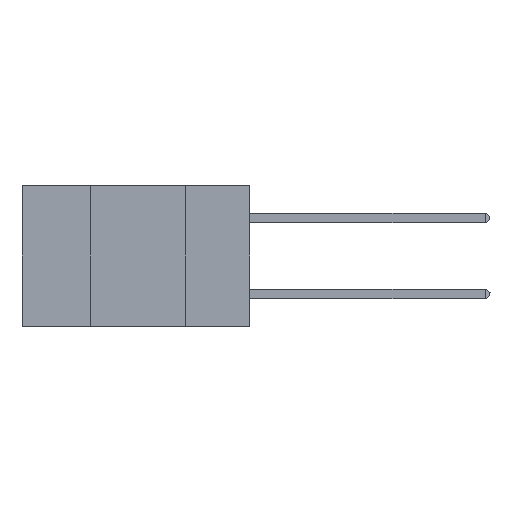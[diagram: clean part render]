
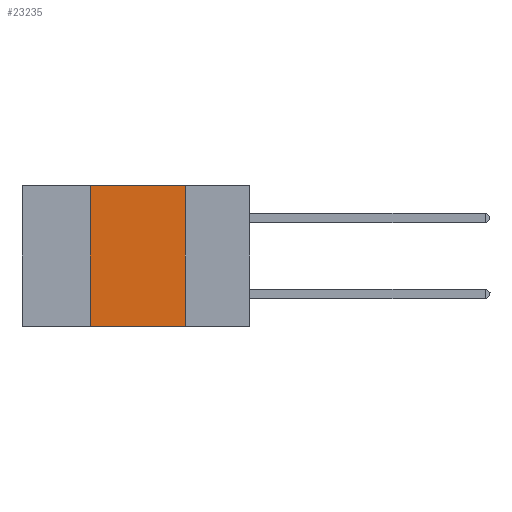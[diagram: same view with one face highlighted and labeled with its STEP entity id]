
A CAD part, left-side view. The second image highlights one B-rep face of the part: STEP entity #23235.
In plain terms, the highlighted planar face has unit normal (-1, 0, 0).
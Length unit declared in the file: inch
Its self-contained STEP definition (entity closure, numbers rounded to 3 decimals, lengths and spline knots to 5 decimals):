
#837 = CARTESIAN_POINT ( 'NONE',  ( 0., 0.42, -0.37 ) ) ;
#2333 = ORIENTED_EDGE ( 'NONE', *, *, #28997, .F. ) ;
#3113 = CARTESIAN_POINT ( 'NONE',  ( 0., 0.6, 0. ) ) ;
#4194 = VERTEX_POINT ( 'NONE', #9329 ) ;
#6163 = PLANE ( 'NONE',  #11271 ) ;
#8453 = ORIENTED_EDGE ( 'NONE', *, *, #9133, .T. ) ;
#9133 = EDGE_CURVE ( 'NONE', #16086, #14528, #12765, .T. ) ;
#9329 = CARTESIAN_POINT ( 'NONE',  ( 0., 0.42, 0. ) ) ;
#10320 = LINE ( 'NONE', #10776, #13405 ) ;
#10776 = CARTESIAN_POINT ( 'NONE',  ( 0., 0.17, 0. ) ) ;
#11271 = AXIS2_PLACEMENT_3D ( 'NONE', #13217, #24995, #15517 ) ;
#11867 = EDGE_CURVE ( 'NONE', #16086, #4194, #12557, .T. ) ;
#12557 = LINE ( 'NONE', #29393, #24395 ) ;
#12635 = VECTOR ( 'NONE', #22107, 39.37008 ) ;
#12765 = LINE ( 'NONE', #26830, #12635 ) ;
#13217 = CARTESIAN_POINT ( 'NONE',  ( 0., 0.6, 0. ) ) ;
#13405 = VECTOR ( 'NONE', #20125, 39.37008 ) ;
#13518 = ORIENTED_EDGE ( 'NONE', *, *, #28529, .F. ) ;
#14528 = VERTEX_POINT ( 'NONE', #24986 ) ;
#15517 = DIRECTION ( 'NONE',  ( 0., 0., -1. ) ) ;
#16086 = VERTEX_POINT ( 'NONE', #837 ) ;
#17223 = DIRECTION ( 'NONE',  ( 0., -1., 0. ) ) ;
#20047 = DIRECTION ( 'NONE',  ( 0., 0., 1. ) ) ;
#20125 = DIRECTION ( 'NONE',  ( 0., 0., -1. ) ) ;
#20560 = FACE_OUTER_BOUND ( 'NONE', #22072, .T. ) ;
#22072 = EDGE_LOOP ( 'NONE', ( #13518, #2333, #29669, #8453 ) ) ;
#22107 = DIRECTION ( 'NONE',  ( 0., -1., 0. ) ) ;
#23235 = ADVANCED_FACE ( 'NONE', ( #20560 ), #6163, .F. ) ;
#24107 = LINE ( 'NONE', #3113, #28563 ) ;
#24395 = VECTOR ( 'NONE', #20047, 39.37008 ) ;
#24986 = CARTESIAN_POINT ( 'NONE',  ( 0., 0.17, -0.37 ) ) ;
#24995 = DIRECTION ( 'NONE',  ( 1., 0., 0. ) ) ;
#25507 = VERTEX_POINT ( 'NONE', #25761 ) ;
#25761 = CARTESIAN_POINT ( 'NONE',  ( 0., 0.17, 0. ) ) ;
#26830 = CARTESIAN_POINT ( 'NONE',  ( 0., 0.6, -0.37 ) ) ;
#28529 = EDGE_CURVE ( 'NONE', #25507, #14528, #10320, .T. ) ;
#28563 = VECTOR ( 'NONE', #17223, 39.37008 ) ;
#28997 = EDGE_CURVE ( 'NONE', #4194, #25507, #24107, .T. ) ;
#29393 = CARTESIAN_POINT ( 'NONE',  ( 0., 0.42, 0. ) ) ;
#29669 = ORIENTED_EDGE ( 'NONE', *, *, #11867, .F. ) ;
